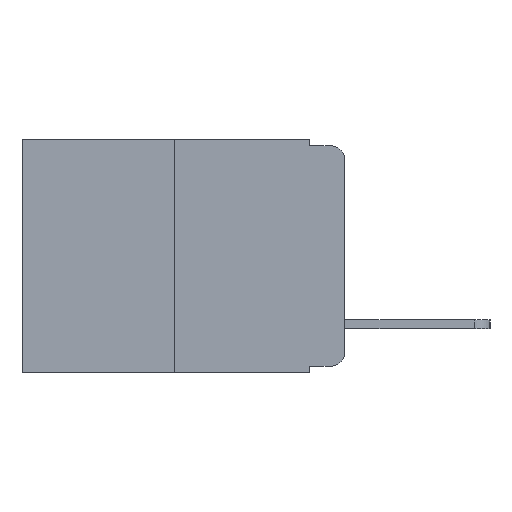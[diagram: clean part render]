
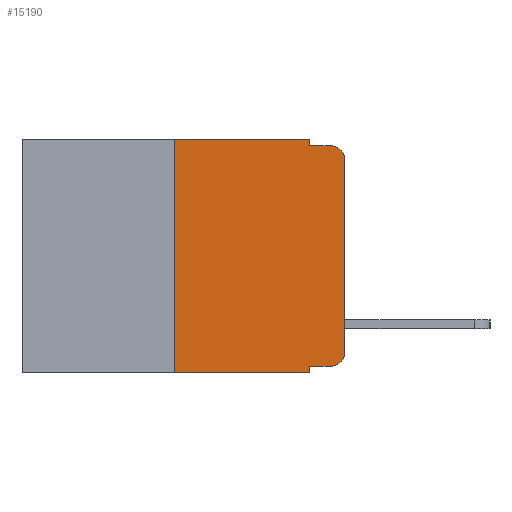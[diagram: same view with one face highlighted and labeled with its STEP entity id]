
A CAD part, left-side view. The second image highlights one B-rep face of the part: STEP entity #15190.
In plain terms, the highlighted planar face has unit normal (-1, 0, 0).
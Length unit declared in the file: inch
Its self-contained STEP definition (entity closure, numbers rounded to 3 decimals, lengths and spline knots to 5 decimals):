
#101 = EDGE_CURVE ( 'NONE', #5992, #11474, #10107, .T. ) ;
#272 = ORIENTED_EDGE ( 'NONE', *, *, #10198, .T. ) ;
#289 = CARTESIAN_POINT ( 'NONE',  ( 0., 0.051, -0.333 ) ) ;
#389 = DIRECTION ( 'NONE',  ( 0., 0., -1. ) ) ;
#1068 = CARTESIAN_POINT ( 'NONE',  ( 0., 0.051, 0. ) ) ;
#1293 = EDGE_CURVE ( 'NONE', #4834, #5992, #19095, .T. ) ;
#1523 = DIRECTION ( 'NONE',  ( 0., -1., 0. ) ) ;
#1631 = ORIENTED_EDGE ( 'NONE', *, *, #3503, .T. ) ;
#2240 = ORIENTED_EDGE ( 'NONE', *, *, #1293, .F. ) ;
#2472 = VERTEX_POINT ( 'NONE', #5915 ) ;
#2513 = CARTESIAN_POINT ( 'NONE',  ( 0., 0.25, 0. ) ) ;
#2525 = EDGE_CURVE ( 'NONE', #13414, #16757, #9481, .T. ) ;
#2846 = DIRECTION ( 'NONE',  ( 0., -1., 0. ) ) ;
#3189 = ORIENTED_EDGE ( 'NONE', *, *, #8953, .T. ) ;
#3331 = ORIENTED_EDGE ( 'NONE', *, *, #5379, .F. ) ;
#3503 = EDGE_CURVE ( 'NONE', #19636, #3587, #16568, .T. ) ;
#3516 = CARTESIAN_POINT ( 'NONE',  ( 0., 0.051, 0. ) ) ;
#3587 = VERTEX_POINT ( 'NONE', #18440 ) ;
#3667 = LINE ( 'NONE', #4581, #15812 ) ;
#3787 = PLANE ( 'NONE',  #7152 ) ;
#3883 = AXIS2_PLACEMENT_3D ( 'NONE', #7462, #18385, #9026 ) ;
#4579 = VERTEX_POINT ( 'NONE', #17059 ) ;
#4581 = CARTESIAN_POINT ( 'NONE',  ( 0., 0.473, -0.343 ) ) ;
#4654 = VERTEX_POINT ( 'NONE', #14179 ) ;
#4669 = ORIENTED_EDGE ( 'NONE', *, *, #2525, .T. ) ;
#4834 = VERTEX_POINT ( 'NONE', #3516 ) ;
#5271 = LINE ( 'NONE', #2513, #17289 ) ;
#5379 = EDGE_CURVE ( 'NONE', #2472, #4579, #5271, .T. ) ;
#5491 = DIRECTION ( 'NONE',  ( 0., -1., 0. ) ) ;
#5740 = AXIS2_PLACEMENT_3D ( 'NONE', #7578, #18490, #9121 ) ;
#5915 = CARTESIAN_POINT ( 'NONE',  ( 0., 0.25, -0.343 ) ) ;
#5992 = VERTEX_POINT ( 'NONE', #11741 ) ;
#6447 = VECTOR ( 'NONE', #1523, 39.37008 ) ;
#6455 = EDGE_CURVE ( 'NONE', #19636, #4654, #15283, .T. ) ;
#6625 = VECTOR ( 'NONE', #14025, 39.37008 ) ;
#7152 = AXIS2_PLACEMENT_3D ( 'NONE', #11807, #10300, #389 ) ;
#7233 = ORIENTED_EDGE ( 'NONE', *, *, #7942, .F. ) ;
#7462 = CARTESIAN_POINT ( 'NONE',  ( 0., 0.02, -0.03 ) ) ;
#7545 = DIRECTION ( 'NONE',  ( 0., 0., 1. ) ) ;
#7578 = CARTESIAN_POINT ( 'NONE',  ( 0., 0.02, -0.313 ) ) ;
#7778 = CARTESIAN_POINT ( 'NONE',  ( 0., 0.02, -0.01 ) ) ;
#7893 = EDGE_LOOP ( 'NONE', ( #4669, #8928, #9889, #2240, #7233, #3331, #272, #7963, #1631, #3189 ) ) ;
#7942 = EDGE_CURVE ( 'NONE', #4579, #4834, #20829, .T. ) ;
#7963 = ORIENTED_EDGE ( 'NONE', *, *, #6455, .F. ) ;
#8057 = EDGE_CURVE ( 'NONE', #16757, #11474, #19884, .T. ) ;
#8928 = ORIENTED_EDGE ( 'NONE', *, *, #8057, .T. ) ;
#8953 = EDGE_CURVE ( 'NONE', #3587, #13414, #19308, .T. ) ;
#9026 = DIRECTION ( 'NONE',  ( 0., 0., -1. ) ) ;
#9121 = DIRECTION ( 'NONE',  ( 0., 0., -1. ) ) ;
#9258 = VECTOR ( 'NONE', #5491, 39.37008 ) ;
#9404 = DIRECTION ( 'NONE',  ( 0., 0., -1. ) ) ;
#9481 = LINE ( 'NONE', #16944, #13618 ) ;
#9889 = ORIENTED_EDGE ( 'NONE', *, *, #101, .F. ) ;
#10107 = LINE ( 'NONE', #19283, #6447 ) ;
#10198 = EDGE_CURVE ( 'NONE', #2472, #4654, #3667, .T. ) ;
#10300 = DIRECTION ( 'NONE',  ( 1., 0., 0. ) ) ;
#10670 = DIRECTION ( 'NONE',  ( 0., 0., 1. ) ) ;
#11474 = VERTEX_POINT ( 'NONE', #7778 ) ;
#11741 = CARTESIAN_POINT ( 'NONE',  ( 0., 0.051, -0.01 ) ) ;
#11807 = CARTESIAN_POINT ( 'NONE',  ( 0., 0.473, 0. ) ) ;
#11870 = DIRECTION ( 'NONE',  ( 0., -1., 0. ) ) ;
#12550 = VECTOR ( 'NONE', #11870, 39.37008 ) ;
#12630 = CARTESIAN_POINT ( 'NONE',  ( 0., 0., -0.03 ) ) ;
#12636 = FACE_OUTER_BOUND ( 'NONE', #7893, .T. ) ;
#13414 = VERTEX_POINT ( 'NONE', #20588 ) ;
#13435 = CARTESIAN_POINT ( 'NONE',  ( 0., 0.473, 0. ) ) ;
#13618 = VECTOR ( 'NONE', #10670, 39.37008 ) ;
#14025 = DIRECTION ( 'NONE',  ( 0., 0., -1. ) ) ;
#14179 = CARTESIAN_POINT ( 'NONE',  ( 0., 0.051, -0.343 ) ) ;
#15190 = ADVANCED_FACE ( 'NONE', ( #12636 ), #3787, .F. ) ;
#15283 = LINE ( 'NONE', #15680, #18983 ) ;
#15680 = CARTESIAN_POINT ( 'NONE',  ( 0., 0.051, 0. ) ) ;
#15812 = VECTOR ( 'NONE', #2846, 39.37008 ) ;
#16568 = LINE ( 'NONE', #289, #9258 ) ;
#16757 = VERTEX_POINT ( 'NONE', #12630 ) ;
#16944 = CARTESIAN_POINT ( 'NONE',  ( 0., 0., 0. ) ) ;
#17059 = CARTESIAN_POINT ( 'NONE',  ( 0., 0.25, 0. ) ) ;
#17289 = VECTOR ( 'NONE', #7545, 39.37008 ) ;
#18385 = DIRECTION ( 'NONE',  ( -1., 0., 0. ) ) ;
#18440 = CARTESIAN_POINT ( 'NONE',  ( 0., 0.02, -0.333 ) ) ;
#18490 = DIRECTION ( 'NONE',  ( -1., 0., 0. ) ) ;
#18983 = VECTOR ( 'NONE', #9404, 39.37008 ) ;
#19095 = LINE ( 'NONE', #1068, #6625 ) ;
#19283 = CARTESIAN_POINT ( 'NONE',  ( 0., 0.051, -0.01 ) ) ;
#19308 = CIRCLE ( 'NONE', #5740, 0.02 ) ;
#19636 = VERTEX_POINT ( 'NONE', #19702 ) ;
#19702 = CARTESIAN_POINT ( 'NONE',  ( 0., 0.051, -0.333 ) ) ;
#19884 = CIRCLE ( 'NONE', #3883, 0.02 ) ;
#20588 = CARTESIAN_POINT ( 'NONE',  ( 0., 0., -0.313 ) ) ;
#20829 = LINE ( 'NONE', #13435, #12550 ) ;
